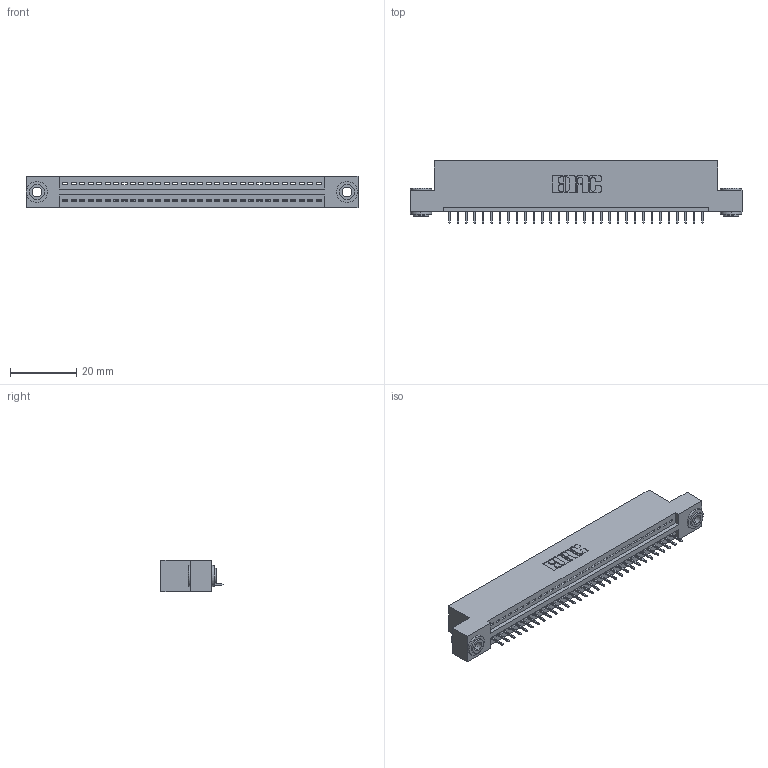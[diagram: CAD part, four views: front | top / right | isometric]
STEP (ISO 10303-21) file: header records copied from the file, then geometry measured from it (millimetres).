
FILE_DESCRIPTION (( 'STEP AP203' ), '1' );
FILE_NAME ('895-031-525-103.STEP', '2020-09-25T18:54:15', ( '' ), ( '' ), 'SwSTEP 2.0', 'SolidWorks 2020', '' );
FILE_SCHEMA (( 'CONFIG_CONTROL_DESIGN' ));
Length unit declared in the file: inch
Products named in the file (4): 345-292-001_345-293-125; 345-250-002_345-250-002-102; 895-031-525-103; 845 Part_Flush Mounting Lugs - 0.156 Dia-TH
Assembly tree (34 placements, depth 2):
  895-031-525-103
    845 Part_Flush Mounting Lugs - 0.156 Dia-TH
    345-292-001_345-293-125  x31
    345-250-002_345-250-002-102  x2
Bounding box: 99.95 x 18.72 x 9.4 mm (x, y, z)
Volume: 9296 mm3; surface area: 11996.4 mm2
Topology: 34 solids, 34 shells, 2086 faces, 5997 edges, 3870 vertices
Faces by surface type: plane 1516, cylinder 562, cone 8
Entity records: 25536 total; most frequent: CARTESIAN_POINT 4400, ORIENTED_EDGE 4358, DIRECTION 3891, EDGE_CURVE 2179, VECTOR 1903, LINE 1903, VERTEX_POINT 1446, AXIS2_PLACEMENT_3D 994
